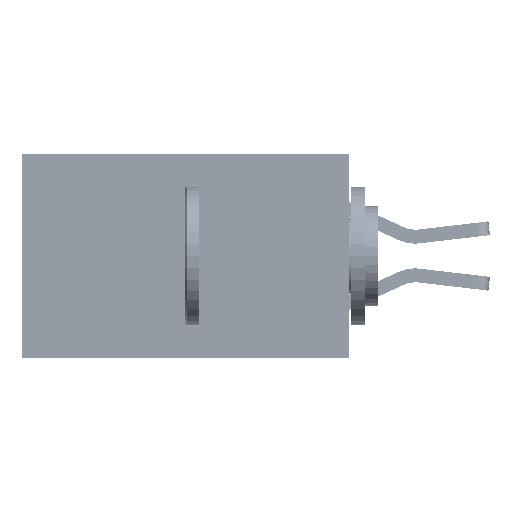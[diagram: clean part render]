
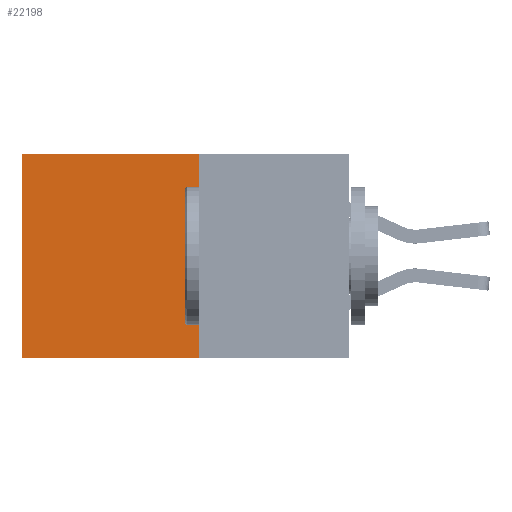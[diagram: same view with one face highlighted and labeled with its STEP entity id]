
A CAD part, left-side view. The second image highlights one B-rep face of the part: STEP entity #22198.
In plain terms, the highlighted planar face has unit normal (-1, 0, 0).
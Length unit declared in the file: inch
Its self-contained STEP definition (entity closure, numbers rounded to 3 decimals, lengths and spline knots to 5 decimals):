
#441 = EDGE_CURVE ( 'NONE', #733, #19527, #27153, .T. ) ;
#733 = VERTEX_POINT ( 'NONE', #15115 ) ;
#1375 = CARTESIAN_POINT ( 'NONE',  ( 0.277, 0.59, -0.37 ) ) ;
#2065 = DIRECTION ( 'NONE',  ( 0., 1., 0. ) ) ;
#2180 = ORIENTED_EDGE ( 'NONE', *, *, #441, .T. ) ;
#2737 = VECTOR ( 'NONE', #30531, 39.37008 ) ;
#3451 = VERTEX_POINT ( 'NONE', #32949 ) ;
#7181 = EDGE_CURVE ( 'NONE', #3451, #19527, #25568, .T. ) ;
#9127 = AXIS2_PLACEMENT_3D ( 'NONE', #13948, #31727, #16577 ) ;
#9491 = EDGE_CURVE ( 'NONE', #17668, #733, #18614, .T. ) ;
#10068 = CARTESIAN_POINT ( 'NONE',  ( 0.277, 0.27, -0.37 ) ) ;
#11669 = EDGE_CURVE ( 'NONE', #17668, #3451, #15634, .T. ) ;
#11705 = VECTOR ( 'NONE', #2065, 39.37008 ) ;
#11856 = VECTOR ( 'NONE', #26586, 39.37008 ) ;
#13803 = DIRECTION ( 'NONE',  ( 0., 0., -1. ) ) ;
#13948 = CARTESIAN_POINT ( 'NONE',  ( 0.277, 0.27, -0.37 ) ) ;
#15115 = CARTESIAN_POINT ( 'NONE',  ( 0.277, 0.59, 0. ) ) ;
#15141 = ORIENTED_EDGE ( 'NONE', *, *, #7181, .F. ) ;
#15634 = LINE ( 'NONE', #10068, #2737 ) ;
#16504 = FACE_OUTER_BOUND ( 'NONE', #28219, .T. ) ;
#16577 = DIRECTION ( 'NONE',  ( 0., 0., -1. ) ) ;
#17668 = VERTEX_POINT ( 'NONE', #24219 ) ;
#18614 = LINE ( 'NONE', #32627, #11705 ) ;
#19527 = VERTEX_POINT ( 'NONE', #1375 ) ;
#21497 = CARTESIAN_POINT ( 'NONE',  ( 0.277, 0.27, -0.37 ) ) ;
#22198 = ADVANCED_FACE ( 'NONE', ( #16504 ), #24204, .F. ) ;
#24204 = PLANE ( 'NONE',  #9127 ) ;
#24219 = CARTESIAN_POINT ( 'NONE',  ( 0.277, 0.27, 0. ) ) ;
#25568 = LINE ( 'NONE', #21497, #11856 ) ;
#26586 = DIRECTION ( 'NONE',  ( 0., 1., 0. ) ) ;
#27153 = LINE ( 'NONE', #29783, #28737 ) ;
#28219 = EDGE_LOOP ( 'NONE', ( #2180, #15141, #32171, #30506 ) ) ;
#28737 = VECTOR ( 'NONE', #13803, 39.37008 ) ;
#29783 = CARTESIAN_POINT ( 'NONE',  ( 0.277, 0.59, -0.37 ) ) ;
#30506 = ORIENTED_EDGE ( 'NONE', *, *, #9491, .T. ) ;
#30531 = DIRECTION ( 'NONE',  ( 0., 0., -1. ) ) ;
#31727 = DIRECTION ( 'NONE',  ( 1., 0., 0. ) ) ;
#32171 = ORIENTED_EDGE ( 'NONE', *, *, #11669, .F. ) ;
#32627 = CARTESIAN_POINT ( 'NONE',  ( 0.277, 0.27, 0. ) ) ;
#32949 = CARTESIAN_POINT ( 'NONE',  ( 0.277, 0.27, -0.37 ) ) ;
